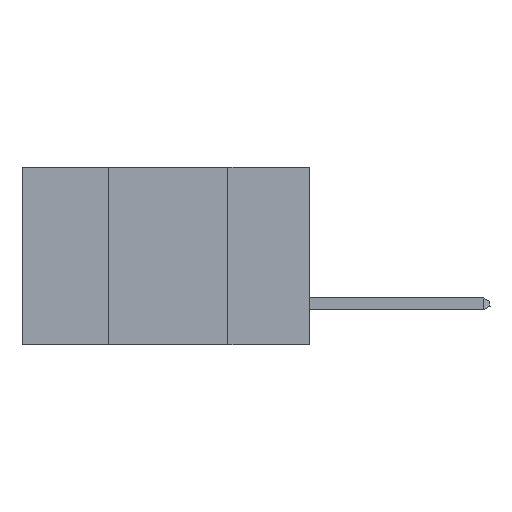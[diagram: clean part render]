
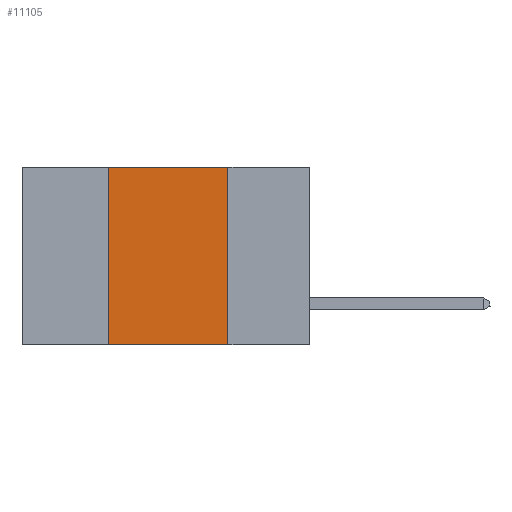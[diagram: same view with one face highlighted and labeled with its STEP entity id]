
A CAD part, left-side view. The second image highlights one B-rep face of the part: STEP entity #11105.
In plain terms, the highlighted planar face has unit normal (-1, 0, 0).
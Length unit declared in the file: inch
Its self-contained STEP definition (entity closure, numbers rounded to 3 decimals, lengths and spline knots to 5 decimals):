
#38 = DIRECTION ( 'NONE',  ( 0., 0., -1. ) ) ;
#606 = VERTEX_POINT ( 'NONE', #14217 ) ;
#1144 = EDGE_CURVE ( 'NONE', #606, #10196, #5540, .T. ) ;
#2905 = LINE ( 'NONE', #5222, #5175 ) ;
#2972 = ORIENTED_EDGE ( 'NONE', *, *, #5088, .T. ) ;
#3318 = CARTESIAN_POINT ( 'NONE',  ( 0., 0.17, -0.37 ) ) ;
#3847 = CARTESIAN_POINT ( 'NONE',  ( 0., 0.6, -0.37 ) ) ;
#3954 = DIRECTION ( 'NONE',  ( 0., -1., 0. ) ) ;
#5088 = EDGE_CURVE ( 'NONE', #13240, #10196, #16287, .T. ) ;
#5175 = VECTOR ( 'NONE', #14432, 39.37008 ) ;
#5222 = CARTESIAN_POINT ( 'NONE',  ( 0., 0.42, 0. ) ) ;
#5249 = DIRECTION ( 'NONE',  ( 0., -1., 0. ) ) ;
#5346 = VECTOR ( 'NONE', #38, 39.37008 ) ;
#5540 = LINE ( 'NONE', #7915, #5346 ) ;
#5585 = FACE_OUTER_BOUND ( 'NONE', #11582, .T. ) ;
#6880 = LINE ( 'NONE', #8762, #15979 ) ;
#7385 = CARTESIAN_POINT ( 'NONE',  ( 0., 0.42, 0. ) ) ;
#7900 = EDGE_CURVE ( 'NONE', #9011, #606, #6880, .T. ) ;
#7915 = CARTESIAN_POINT ( 'NONE',  ( 0., 0.17, 0. ) ) ;
#8628 = VECTOR ( 'NONE', #5249, 39.37008 ) ;
#8762 = CARTESIAN_POINT ( 'NONE',  ( 0., 0.6, 0. ) ) ;
#9011 = VERTEX_POINT ( 'NONE', #7385 ) ;
#9900 = AXIS2_PLACEMENT_3D ( 'NONE', #11581, #15588, #16842 ) ;
#10196 = VERTEX_POINT ( 'NONE', #3318 ) ;
#11105 = ADVANCED_FACE ( 'NONE', ( #5585 ), #16664, .F. ) ;
#11130 = ORIENTED_EDGE ( 'NONE', *, *, #7900, .F. ) ;
#11581 = CARTESIAN_POINT ( 'NONE',  ( 0., 0.6, 0. ) ) ;
#11582 = EDGE_LOOP ( 'NONE', ( #13564, #11130, #14748, #2972 ) ) ;
#13240 = VERTEX_POINT ( 'NONE', #14179 ) ;
#13564 = ORIENTED_EDGE ( 'NONE', *, *, #1144, .F. ) ;
#14179 = CARTESIAN_POINT ( 'NONE',  ( 0., 0.42, -0.37 ) ) ;
#14217 = CARTESIAN_POINT ( 'NONE',  ( 0., 0.17, 0. ) ) ;
#14432 = DIRECTION ( 'NONE',  ( 0., 0., 1. ) ) ;
#14748 = ORIENTED_EDGE ( 'NONE', *, *, #15329, .F. ) ;
#15329 = EDGE_CURVE ( 'NONE', #13240, #9011, #2905, .T. ) ;
#15588 = DIRECTION ( 'NONE',  ( 1., 0., 0. ) ) ;
#15979 = VECTOR ( 'NONE', #3954, 39.37008 ) ;
#16287 = LINE ( 'NONE', #3847, #8628 ) ;
#16664 = PLANE ( 'NONE',  #9900 ) ;
#16842 = DIRECTION ( 'NONE',  ( 0., 0., -1. ) ) ;
